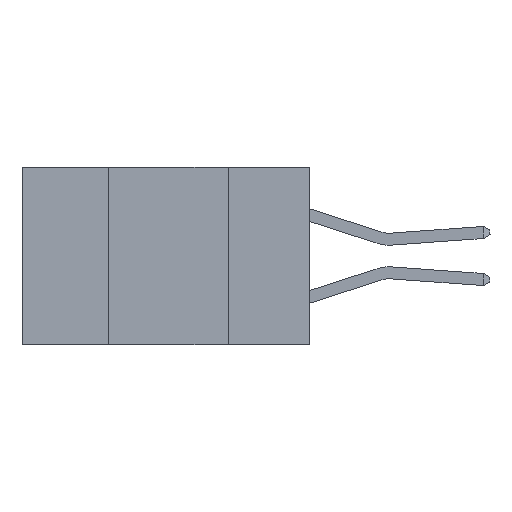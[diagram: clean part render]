
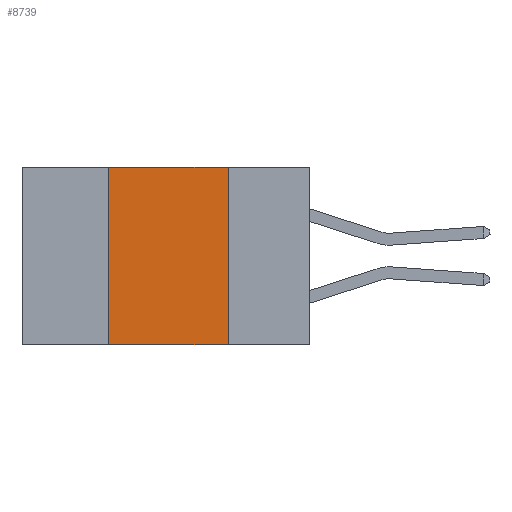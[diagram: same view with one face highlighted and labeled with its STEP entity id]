
A CAD part, left-side view. The second image highlights one B-rep face of the part: STEP entity #8739.
In plain terms, the highlighted planar face has unit normal (-1, 0, 0).
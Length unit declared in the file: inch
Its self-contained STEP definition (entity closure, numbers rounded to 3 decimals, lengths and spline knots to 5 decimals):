
#2150 = CARTESIAN_POINT ( 'NONE',  ( 0., 0.6, 0. ) ) ;
#3486 = LINE ( 'NONE', #18033, #16819 ) ;
#4262 = PLANE ( 'NONE',  #6828 ) ;
#4579 = DIRECTION ( 'NONE',  ( 0., 0., 1. ) ) ;
#5275 = CARTESIAN_POINT ( 'NONE',  ( 0., 0.17, 0. ) ) ;
#5365 = LINE ( 'NONE', #23230, #21417 ) ;
#5467 = EDGE_CURVE ( 'NONE', #6290, #6945, #22129, .T. ) ;
#6290 = VERTEX_POINT ( 'NONE', #19040 ) ;
#6460 = DIRECTION ( 'NONE',  ( 0., -1., 0. ) ) ;
#6828 = AXIS2_PLACEMENT_3D ( 'NONE', #2150, #15914, #19824 ) ;
#6945 = VERTEX_POINT ( 'NONE', #13442 ) ;
#7842 = DIRECTION ( 'NONE',  ( 0., -1., 0. ) ) ;
#8080 = ORIENTED_EDGE ( 'NONE', *, *, #17463, .T. ) ;
#8739 = ADVANCED_FACE ( 'NONE', ( #10448 ), #4262, .F. ) ;
#9791 = CARTESIAN_POINT ( 'NONE',  ( 0., 0.6, 0. ) ) ;
#10355 = CARTESIAN_POINT ( 'NONE',  ( 0., 0.42, 0. ) ) ;
#10448 = FACE_OUTER_BOUND ( 'NONE', #17969, .T. ) ;
#11643 = DIRECTION ( 'NONE',  ( 0., 0., -1. ) ) ;
#11816 = VERTEX_POINT ( 'NONE', #5275 ) ;
#12821 = ORIENTED_EDGE ( 'NONE', *, *, #5467, .F. ) ;
#13442 = CARTESIAN_POINT ( 'NONE',  ( 0., 0.42, 0. ) ) ;
#15115 = EDGE_CURVE ( 'NONE', #6945, #11816, #18282, .T. ) ;
#15914 = DIRECTION ( 'NONE',  ( 1., 0., 0. ) ) ;
#16819 = VECTOR ( 'NONE', #6460, 39.37008 ) ;
#17463 = EDGE_CURVE ( 'NONE', #6290, #24938, #3486, .T. ) ;
#17969 = EDGE_LOOP ( 'NONE', ( #18748, #25010, #12821, #8080 ) ) ;
#18033 = CARTESIAN_POINT ( 'NONE',  ( 0., 0.6, -0.37 ) ) ;
#18282 = LINE ( 'NONE', #9791, #21368 ) ;
#18748 = ORIENTED_EDGE ( 'NONE', *, *, #21824, .F. ) ;
#19040 = CARTESIAN_POINT ( 'NONE',  ( 0., 0.42, -0.37 ) ) ;
#19824 = DIRECTION ( 'NONE',  ( 0., 0., -1. ) ) ;
#20945 = CARTESIAN_POINT ( 'NONE',  ( 0., 0.17, -0.37 ) ) ;
#21368 = VECTOR ( 'NONE', #7842, 39.37008 ) ;
#21417 = VECTOR ( 'NONE', #11643, 39.37008 ) ;
#21824 = EDGE_CURVE ( 'NONE', #11816, #24938, #5365, .T. ) ;
#22129 = LINE ( 'NONE', #10355, #23317 ) ;
#23230 = CARTESIAN_POINT ( 'NONE',  ( 0., 0.17, 0. ) ) ;
#23317 = VECTOR ( 'NONE', #4579, 39.37008 ) ;
#24938 = VERTEX_POINT ( 'NONE', #20945 ) ;
#25010 = ORIENTED_EDGE ( 'NONE', *, *, #15115, .F. ) ;
